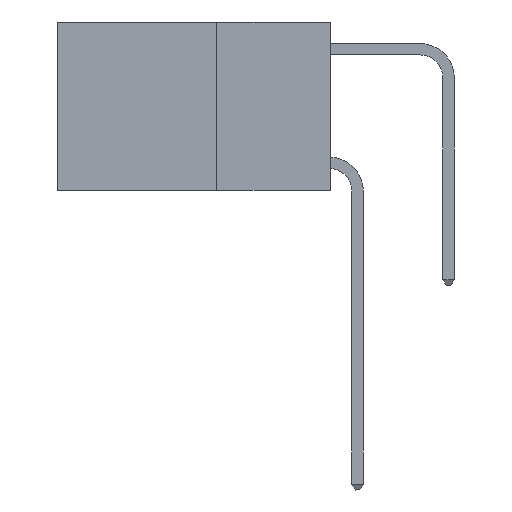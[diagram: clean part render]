
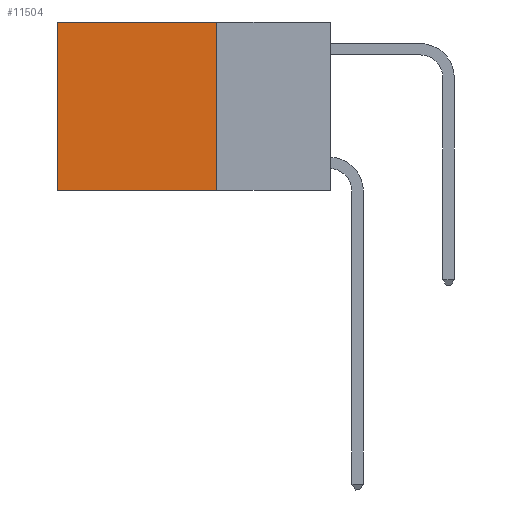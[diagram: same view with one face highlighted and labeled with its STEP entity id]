
A CAD part, left-side view. The second image highlights one B-rep face of the part: STEP entity #11504.
In plain terms, the highlighted planar face has unit normal (-1, 0, 0).
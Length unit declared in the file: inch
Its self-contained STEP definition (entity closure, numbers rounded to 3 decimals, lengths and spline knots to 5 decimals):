
#87 = DIRECTION ( 'NONE',  ( 0., 0., -1. ) ) ;
#138 = CARTESIAN_POINT ( 'NONE',  ( 0.2625, 0.25, 0. ) ) ;
#321 = LINE ( 'NONE', #9227, #910 ) ;
#824 = DIRECTION ( 'NONE',  ( 0., 1., 0. ) ) ;
#910 = VECTOR ( 'NONE', #3880, 39.37008 ) ;
#1410 = ORIENTED_EDGE ( 'NONE', *, *, #2596, .F. ) ;
#1560 = VECTOR ( 'NONE', #10538, 39.37008 ) ;
#1805 = VERTEX_POINT ( 'NONE', #10201 ) ;
#2596 = EDGE_CURVE ( 'NONE', #6979, #1805, #321, .T. ) ;
#3023 = CARTESIAN_POINT ( 'NONE',  ( 0.2625, 0.6, -0.37 ) ) ;
#3234 = EDGE_CURVE ( 'NONE', #8886, #5957, #7847, .T. ) ;
#3880 = DIRECTION ( 'NONE',  ( 0., 0., -1. ) ) ;
#4577 = VECTOR ( 'NONE', #824, 39.37008 ) ;
#5176 = CARTESIAN_POINT ( 'NONE',  ( 0.2625, 0.6, 0. ) ) ;
#5407 = ORIENTED_EDGE ( 'NONE', *, *, #6729, .T. ) ;
#5957 = VERTEX_POINT ( 'NONE', #3023 ) ;
#6016 = FACE_OUTER_BOUND ( 'NONE', #7383, .T. ) ;
#6075 = CARTESIAN_POINT ( 'NONE',  ( 0.2625, 0.6, 0. ) ) ;
#6131 = DIRECTION ( 'NONE',  ( 1., 0., 0. ) ) ;
#6729 = EDGE_CURVE ( 'NONE', #6979, #8886, #9909, .T. ) ;
#6979 = VERTEX_POINT ( 'NONE', #9324 ) ;
#7067 = AXIS2_PLACEMENT_3D ( 'NONE', #11389, #6131, #87 ) ;
#7383 = EDGE_LOOP ( 'NONE', ( #8773, #10360, #1410, #5407 ) ) ;
#7675 = LINE ( 'NONE', #11248, #10404 ) ;
#7847 = LINE ( 'NONE', #5176, #1560 ) ;
#8773 = ORIENTED_EDGE ( 'NONE', *, *, #3234, .T. ) ;
#8886 = VERTEX_POINT ( 'NONE', #6075 ) ;
#9221 = EDGE_CURVE ( 'NONE', #1805, #5957, #7675, .T. ) ;
#9227 = CARTESIAN_POINT ( 'NONE',  ( 0.2625, 0.25, 0. ) ) ;
#9324 = CARTESIAN_POINT ( 'NONE',  ( 0.2625, 0.25, 0. ) ) ;
#9744 = PLANE ( 'NONE',  #7067 ) ;
#9909 = LINE ( 'NONE', #138, #4577 ) ;
#10201 = CARTESIAN_POINT ( 'NONE',  ( 0.2625, 0.25, -0.37 ) ) ;
#10360 = ORIENTED_EDGE ( 'NONE', *, *, #9221, .F. ) ;
#10363 = DIRECTION ( 'NONE',  ( 0., 1., 0. ) ) ;
#10404 = VECTOR ( 'NONE', #10363, 39.37008 ) ;
#10538 = DIRECTION ( 'NONE',  ( 0., 0., -1. ) ) ;
#11248 = CARTESIAN_POINT ( 'NONE',  ( 0.2625, 0.25, -0.37 ) ) ;
#11389 = CARTESIAN_POINT ( 'NONE',  ( 0.2625, 0.25, 0. ) ) ;
#11504 = ADVANCED_FACE ( 'NONE', ( #6016 ), #9744, .F. ) ;
